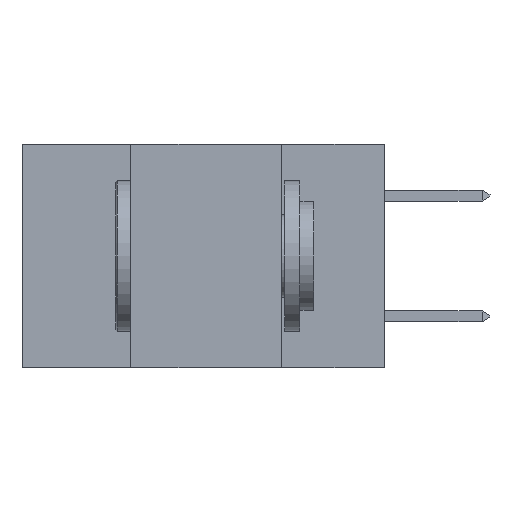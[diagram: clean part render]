
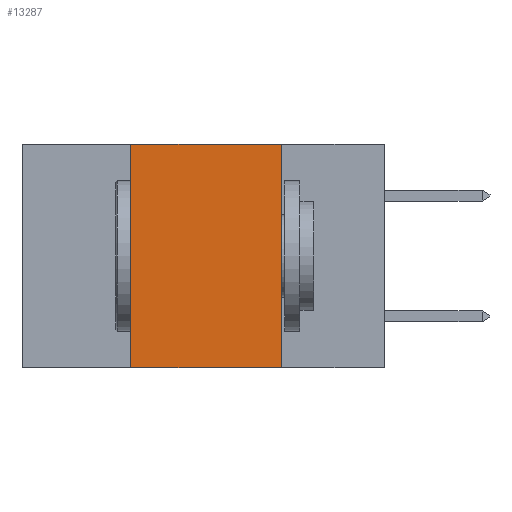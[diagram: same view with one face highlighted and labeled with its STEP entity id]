
A CAD part, left-side view. The second image highlights one B-rep face of the part: STEP entity #13287.
In plain terms, the highlighted planar face has unit normal (-1, 0, 0).
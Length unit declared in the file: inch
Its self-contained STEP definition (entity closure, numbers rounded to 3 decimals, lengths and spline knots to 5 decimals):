
#308 = DIRECTION ( 'NONE',  ( 1., 0., 0. ) ) ;
#1062 = VERTEX_POINT ( 'NONE', #22150 ) ;
#1181 = CARTESIAN_POINT ( 'NONE',  ( 0., 0.17, 0. ) ) ;
#1561 = ORIENTED_EDGE ( 'NONE', *, *, #1921, .F. ) ;
#1921 = EDGE_CURVE ( 'NONE', #1062, #19402, #5548, .T. ) ;
#2667 = LINE ( 'NONE', #22582, #23506 ) ;
#3508 = ORIENTED_EDGE ( 'NONE', *, *, #3582, .T. ) ;
#3582 = EDGE_CURVE ( 'NONE', #1062, #7692, #2667, .T. ) ;
#3873 = DIRECTION ( 'NONE',  ( 0., -1., 0. ) ) ;
#4665 = VECTOR ( 'NONE', #22216, 39.37008 ) ;
#4920 = VECTOR ( 'NONE', #18745, 39.37008 ) ;
#5285 = LINE ( 'NONE', #20297, #4665 ) ;
#5548 = LINE ( 'NONE', #17730, #4920 ) ;
#7692 = VERTEX_POINT ( 'NONE', #14021 ) ;
#9312 = EDGE_LOOP ( 'NONE', ( #15247, #18306, #1561, #3508 ) ) ;
#10883 = EDGE_CURVE ( 'NONE', #19402, #19114, #16465, .T. ) ;
#12091 = PLANE ( 'NONE',  #18688 ) ;
#13287 = ADVANCED_FACE ( 'NONE', ( #25220 ), #12091, .F. ) ;
#14021 = CARTESIAN_POINT ( 'NONE',  ( 0., 0.17, -0.37 ) ) ;
#14068 = DIRECTION ( 'NONE',  ( 0., 0., -1. ) ) ;
#15247 = ORIENTED_EDGE ( 'NONE', *, *, #25233, .F. ) ;
#15876 = CARTESIAN_POINT ( 'NONE',  ( 0., 0.42, 0. ) ) ;
#16465 = LINE ( 'NONE', #17573, #21051 ) ;
#17573 = CARTESIAN_POINT ( 'NONE',  ( 0., 0.6, 0. ) ) ;
#17730 = CARTESIAN_POINT ( 'NONE',  ( 0., 0.42, 0. ) ) ;
#17980 = CARTESIAN_POINT ( 'NONE',  ( 0., 0.6, 0. ) ) ;
#18306 = ORIENTED_EDGE ( 'NONE', *, *, #10883, .F. ) ;
#18688 = AXIS2_PLACEMENT_3D ( 'NONE', #17980, #308, #14068 ) ;
#18745 = DIRECTION ( 'NONE',  ( 0., 0., 1. ) ) ;
#19114 = VERTEX_POINT ( 'NONE', #1181 ) ;
#19402 = VERTEX_POINT ( 'NONE', #15876 ) ;
#20297 = CARTESIAN_POINT ( 'NONE',  ( 0., 0.17, 0. ) ) ;
#21051 = VECTOR ( 'NONE', #3873, 39.37008 ) ;
#22150 = CARTESIAN_POINT ( 'NONE',  ( 0., 0.42, -0.37 ) ) ;
#22216 = DIRECTION ( 'NONE',  ( 0., 0., -1. ) ) ;
#22582 = CARTESIAN_POINT ( 'NONE',  ( 0., 0.6, -0.37 ) ) ;
#23506 = VECTOR ( 'NONE', #24005, 39.37008 ) ;
#24005 = DIRECTION ( 'NONE',  ( 0., -1., 0. ) ) ;
#25220 = FACE_OUTER_BOUND ( 'NONE', #9312, .T. ) ;
#25233 = EDGE_CURVE ( 'NONE', #19114, #7692, #5285, .T. ) ;
